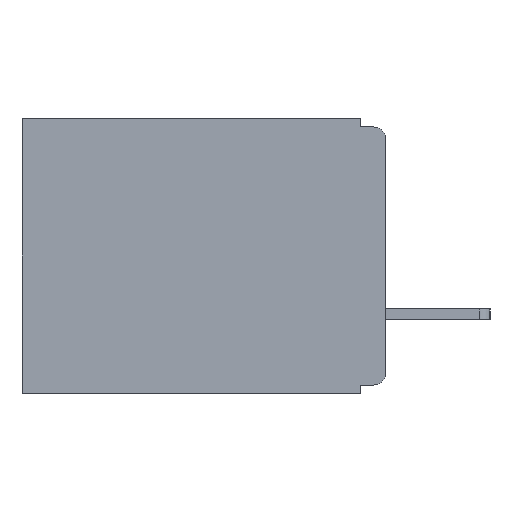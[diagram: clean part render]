
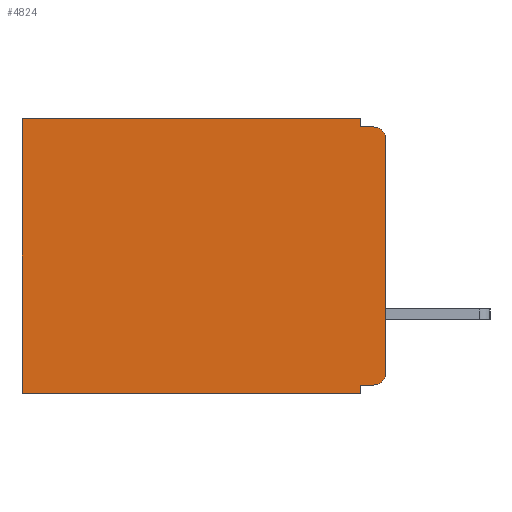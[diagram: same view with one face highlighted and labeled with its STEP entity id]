
A CAD part, left-side view. The second image highlights one B-rep face of the part: STEP entity #4824.
In plain terms, the highlighted planar face has unit normal (-1, 0, 0).
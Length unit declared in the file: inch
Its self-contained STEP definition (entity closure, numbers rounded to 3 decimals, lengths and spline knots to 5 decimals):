
#1144 = PLANE ( 'NONE',  #3606 ) ;
#2085 = DIRECTION ( 'NONE',  ( 0., 0., -1. ) ) ;
#2403 = DIRECTION ( 'NONE',  ( 0., 1., 0. ) ) ;
#2454 = CARTESIAN_POINT ( 'NONE',  ( 0.3, 0.015, -0.01 ) ) ;
#2695 = CARTESIAN_POINT ( 'NONE',  ( 0.3, 0., -0.33 ) ) ;
#3273 = LINE ( 'NONE', #3385, #10549 ) ;
#3291 = EDGE_CURVE ( 'NONE', #15969, #5419, #11067, .T. ) ;
#3385 = CARTESIAN_POINT ( 'NONE',  ( 0.3, 0., -0.33 ) ) ;
#3424 = ORIENTED_EDGE ( 'NONE', *, *, #18217, .F. ) ;
#3466 = DIRECTION ( 'NONE',  ( 0., -1., 0. ) ) ;
#3529 = CARTESIAN_POINT ( 'NONE',  ( 0.3, 0., -0.01 ) ) ;
#3599 = LINE ( 'NONE', #5166, #9539 ) ;
#3606 = AXIS2_PLACEMENT_3D ( 'NONE', #2695, #4049, #4025 ) ;
#3610 = DIRECTION ( 'NONE',  ( 0., 1., 0. ) ) ;
#3630 = VECTOR ( 'NONE', #3610, 39.37008 ) ;
#3736 = FACE_OUTER_BOUND ( 'NONE', #10393, .T. ) ;
#3985 = DIRECTION ( 'NONE',  ( 0., 0., -1. ) ) ;
#4025 = DIRECTION ( 'NONE',  ( 0., 0., -1. ) ) ;
#4049 = DIRECTION ( 'NONE',  ( 1., 0., 0. ) ) ;
#4567 = EDGE_CURVE ( 'NONE', #10269, #16632, #15163, .T. ) ;
#4647 = ORIENTED_EDGE ( 'NONE', *, *, #3291, .T. ) ;
#4709 = LINE ( 'NONE', #5242, #8127 ) ;
#4729 = EDGE_CURVE ( 'NONE', #9611, #15969, #16295, .T. ) ;
#4824 = ADVANCED_FACE ( 'NONE', ( #3736 ), #1144, .F. ) ;
#4829 = EDGE_CURVE ( 'NONE', #13033, #16632, #3273, .T. ) ;
#5166 = CARTESIAN_POINT ( 'NONE',  ( 0.3, 0.031, -0.33 ) ) ;
#5242 = CARTESIAN_POINT ( 'NONE',  ( 0.3, 0.031, 0. ) ) ;
#5419 = VERTEX_POINT ( 'NONE', #16301 ) ;
#5659 = DIRECTION ( 'NONE',  ( -1., 0., 0. ) ) ;
#5842 = CARTESIAN_POINT ( 'NONE',  ( 0.3, 0.031, -0.32 ) ) ;
#5917 = AXIS2_PLACEMENT_3D ( 'NONE', #16130, #5659, #12507 ) ;
#6271 = VERTEX_POINT ( 'NONE', #9563 ) ;
#6308 = DIRECTION ( 'NONE',  ( -1., 0., 0. ) ) ;
#6348 = CARTESIAN_POINT ( 'NONE',  ( 0.3, 0.015, -0.32 ) ) ;
#7136 = ORIENTED_EDGE ( 'NONE', *, *, #14549, .F. ) ;
#7196 = VECTOR ( 'NONE', #2085, 39.37008 ) ;
#7345 = EDGE_CURVE ( 'NONE', #6271, #5419, #14346, .T. ) ;
#7679 = VECTOR ( 'NONE', #3466, 39.37008 ) ;
#8127 = VECTOR ( 'NONE', #12436, 39.37008 ) ;
#8920 = VECTOR ( 'NONE', #2403, 39.37008 ) ;
#8973 = AXIS2_PLACEMENT_3D ( 'NONE', #15074, #6308, #16542 ) ;
#9045 = CARTESIAN_POINT ( 'NONE',  ( 0.3, 0.031, -0.01 ) ) ;
#9078 = EDGE_CURVE ( 'NONE', #11902, #9207, #15475, .T. ) ;
#9207 = VERTEX_POINT ( 'NONE', #2454 ) ;
#9438 = ORIENTED_EDGE ( 'NONE', *, *, #15558, .F. ) ;
#9539 = VECTOR ( 'NONE', #13923, 39.37008 ) ;
#9563 = CARTESIAN_POINT ( 'NONE',  ( 0.3, 0.031, -0.33 ) ) ;
#9611 = VERTEX_POINT ( 'NONE', #14944 ) ;
#9667 = ORIENTED_EDGE ( 'NONE', *, *, #11368, .T. ) ;
#10269 = VERTEX_POINT ( 'NONE', #6348 ) ;
#10325 = ORIENTED_EDGE ( 'NONE', *, *, #9078, .F. ) ;
#10393 = EDGE_LOOP ( 'NONE', ( #12892, #9667, #10325, #9438, #11892, #4647, #13977, #7136, #3424, #16061 ) ) ;
#10519 = CARTESIAN_POINT ( 'NONE',  ( 0.3, 0.437, 0. ) ) ;
#10549 = VECTOR ( 'NONE', #3985, 39.37008 ) ;
#11067 = LINE ( 'NONE', #13765, #7196 ) ;
#11368 = EDGE_CURVE ( 'NONE', #13033, #9207, #15384, .T. ) ;
#11631 = CARTESIAN_POINT ( 'NONE',  ( 0.3, 0., 0. ) ) ;
#11892 = ORIENTED_EDGE ( 'NONE', *, *, #4729, .T. ) ;
#11902 = VERTEX_POINT ( 'NONE', #9045 ) ;
#12365 = VECTOR ( 'NONE', #12700, 39.37008 ) ;
#12436 = DIRECTION ( 'NONE',  ( 0., 0., -1. ) ) ;
#12507 = DIRECTION ( 'NONE',  ( 0., 0., -1. ) ) ;
#12700 = DIRECTION ( 'NONE',  ( 0., 1., 0. ) ) ;
#12892 = ORIENTED_EDGE ( 'NONE', *, *, #4829, .F. ) ;
#13033 = VERTEX_POINT ( 'NONE', #16223 ) ;
#13509 = CARTESIAN_POINT ( 'NONE',  ( 0.3, 0., -0.305 ) ) ;
#13765 = CARTESIAN_POINT ( 'NONE',  ( 0.3, 0.437, -0.33 ) ) ;
#13923 = DIRECTION ( 'NONE',  ( 0., 0., -1. ) ) ;
#13977 = ORIENTED_EDGE ( 'NONE', *, *, #7345, .F. ) ;
#14004 = CARTESIAN_POINT ( 'NONE',  ( 0.3, 0., -0.32 ) ) ;
#14346 = LINE ( 'NONE', #16702, #3630 ) ;
#14549 = EDGE_CURVE ( 'NONE', #17572, #6271, #3599, .T. ) ;
#14944 = CARTESIAN_POINT ( 'NONE',  ( 0.3, 0.031, 0. ) ) ;
#15074 = CARTESIAN_POINT ( 'NONE',  ( 0.3, 0.015, -0.025 ) ) ;
#15163 = CIRCLE ( 'NONE', #5917, 0.015 ) ;
#15384 = CIRCLE ( 'NONE', #8973, 0.015 ) ;
#15475 = LINE ( 'NONE', #3529, #7679 ) ;
#15558 = EDGE_CURVE ( 'NONE', #9611, #11902, #4709, .T. ) ;
#15969 = VERTEX_POINT ( 'NONE', #10519 ) ;
#16061 = ORIENTED_EDGE ( 'NONE', *, *, #4567, .T. ) ;
#16130 = CARTESIAN_POINT ( 'NONE',  ( 0.3, 0.015, -0.305 ) ) ;
#16223 = CARTESIAN_POINT ( 'NONE',  ( 0.3, 0., -0.025 ) ) ;
#16295 = LINE ( 'NONE', #11631, #12365 ) ;
#16301 = CARTESIAN_POINT ( 'NONE',  ( 0.3, 0.437, -0.33 ) ) ;
#16542 = DIRECTION ( 'NONE',  ( 0., 0., -1. ) ) ;
#16632 = VERTEX_POINT ( 'NONE', #13509 ) ;
#16702 = CARTESIAN_POINT ( 'NONE',  ( 0.3, 0., -0.33 ) ) ;
#16706 = LINE ( 'NONE', #14004, #8920 ) ;
#17572 = VERTEX_POINT ( 'NONE', #5842 ) ;
#18217 = EDGE_CURVE ( 'NONE', #10269, #17572, #16706, .T. ) ;
